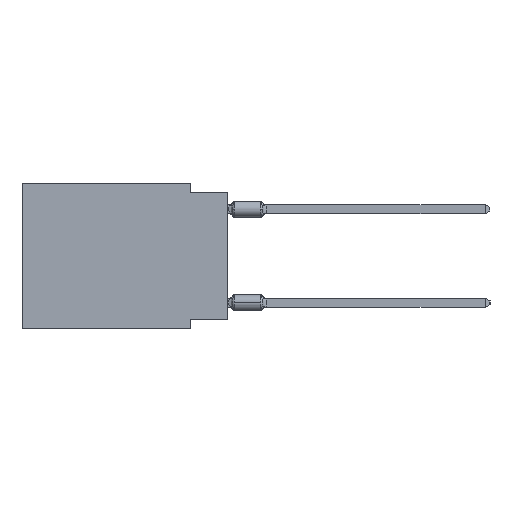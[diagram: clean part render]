
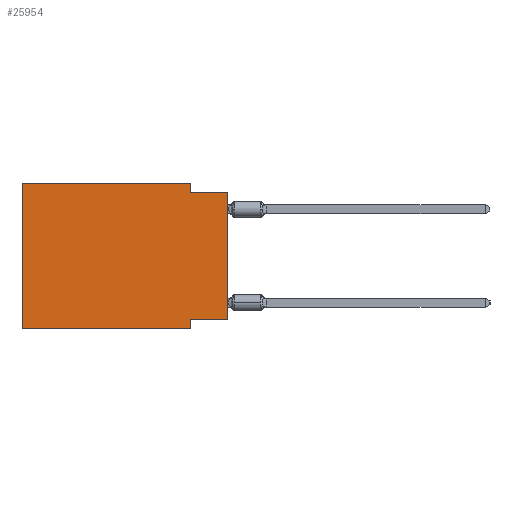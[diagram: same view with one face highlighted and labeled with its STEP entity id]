
A CAD part, left-side view. The second image highlights one B-rep face of the part: STEP entity #25954.
In plain terms, the highlighted planar face has unit normal (-1, 0, 0).
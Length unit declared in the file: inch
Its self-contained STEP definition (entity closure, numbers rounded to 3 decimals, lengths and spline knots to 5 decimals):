
#941 = ORIENTED_EDGE ( 'NONE', *, *, #7162, .T. ) ;
#1256 = EDGE_CURVE ( 'NONE', #4741, #25546, #44619, .T. ) ;
#1490 = LINE ( 'NONE', #14653, #12118 ) ;
#1783 = DIRECTION ( 'NONE',  ( 0., -1., 0. ) ) ;
#2938 = VECTOR ( 'NONE', #43295, 39.37008 ) ;
#3073 = LINE ( 'NONE', #11270, #56207 ) ;
#4071 = VERTEX_POINT ( 'NONE', #52990 ) ;
#4741 = VERTEX_POINT ( 'NONE', #26559 ) ;
#5107 = CARTESIAN_POINT ( 'NONE',  ( 0., 0.1, -0.025 ) ) ;
#7162 = EDGE_CURVE ( 'NONE', #4741, #17069, #37907, .T. ) ;
#7419 = CARTESIAN_POINT ( 'NONE',  ( 0., 0., -0.025 ) ) ;
#7439 = ORIENTED_EDGE ( 'NONE', *, *, #41969, .F. ) ;
#8390 = VECTOR ( 'NONE', #41917, 39.37008 ) ;
#10567 = LINE ( 'NONE', #11135, #43037 ) ;
#10847 = DIRECTION ( 'NONE',  ( 0., 0., 1. ) ) ;
#11135 = CARTESIAN_POINT ( 'NONE',  ( 0., 0., -0.365 ) ) ;
#11270 = CARTESIAN_POINT ( 'NONE',  ( 0., 0.55, 0. ) ) ;
#12118 = VECTOR ( 'NONE', #1783, 39.37008 ) ;
#12351 = CARTESIAN_POINT ( 'NONE',  ( 0., 0.1, -0.39 ) ) ;
#14587 = FACE_OUTER_BOUND ( 'NONE', #33785, .T. ) ;
#14653 = CARTESIAN_POINT ( 'NONE',  ( 0., 0., -0.025 ) ) ;
#15165 = CARTESIAN_POINT ( 'NONE',  ( 0., 0.55, 0. ) ) ;
#17069 = VERTEX_POINT ( 'NONE', #12351 ) ;
#20062 = ORIENTED_EDGE ( 'NONE', *, *, #33660, .T. ) ;
#20437 = LINE ( 'NONE', #38310, #2938 ) ;
#20591 = EDGE_CURVE ( 'NONE', #52373, #43440, #1490, .T. ) ;
#21162 = ORIENTED_EDGE ( 'NONE', *, *, #32842, .F. ) ;
#21853 = EDGE_CURVE ( 'NONE', #40993, #4071, #10567, .T. ) ;
#22333 = CARTESIAN_POINT ( 'NONE',  ( 0., 0.55, 0. ) ) ;
#24034 = LINE ( 'NONE', #37512, #8390 ) ;
#25017 = DIRECTION ( 'NONE',  ( 0., -1., 0. ) ) ;
#25546 = VERTEX_POINT ( 'NONE', #28119 ) ;
#25954 = ADVANCED_FACE ( 'NONE', ( #14587 ), #50323, .F. ) ;
#26559 = CARTESIAN_POINT ( 'NONE',  ( 0., 0.55, -0.39 ) ) ;
#28119 = CARTESIAN_POINT ( 'NONE',  ( 0., 0.55, 0. ) ) ;
#28281 = ORIENTED_EDGE ( 'NONE', *, *, #1256, .F. ) ;
#28833 = DIRECTION ( 'NONE',  ( 0., -1., 0. ) ) ;
#30978 = CARTESIAN_POINT ( 'NONE',  ( 0., 0., -0.365 ) ) ;
#32842 = EDGE_CURVE ( 'NONE', #25546, #52557, #3073, .T. ) ;
#33028 = DIRECTION ( 'NONE',  ( 1., 0., 0. ) ) ;
#33385 = CARTESIAN_POINT ( 'NONE',  ( 0., 0., 0. ) ) ;
#33660 = EDGE_CURVE ( 'NONE', #40993, #43440, #42461, .T. ) ;
#33785 = EDGE_LOOP ( 'NONE', ( #20062, #37670, #7439, #21162, #28281, #941, #42858, #34050 ) ) ;
#33812 = CARTESIAN_POINT ( 'NONE',  ( 0., 0.55, -0.39 ) ) ;
#33816 = VECTOR ( 'NONE', #10847, 39.37008 ) ;
#34050 = ORIENTED_EDGE ( 'NONE', *, *, #21853, .F. ) ;
#34061 = CARTESIAN_POINT ( 'NONE',  ( 0., 0.1, 0. ) ) ;
#34201 = VECTOR ( 'NONE', #25017, 39.37008 ) ;
#37512 = CARTESIAN_POINT ( 'NONE',  ( 0., 0.1, 0. ) ) ;
#37670 = ORIENTED_EDGE ( 'NONE', *, *, #20591, .F. ) ;
#37907 = LINE ( 'NONE', #33812, #34201 ) ;
#38310 = CARTESIAN_POINT ( 'NONE',  ( 0., 0.1, -0.39 ) ) ;
#40993 = VERTEX_POINT ( 'NONE', #30978 ) ;
#41917 = DIRECTION ( 'NONE',  ( 0., 0., -1. ) ) ;
#41969 = EDGE_CURVE ( 'NONE', #52557, #52373, #24034, .T. ) ;
#42461 = LINE ( 'NONE', #33385, #33816 ) ;
#42858 = ORIENTED_EDGE ( 'NONE', *, *, #46620, .F. ) ;
#43037 = VECTOR ( 'NONE', #46280, 39.37008 ) ;
#43295 = DIRECTION ( 'NONE',  ( 0., 0., -1. ) ) ;
#43440 = VERTEX_POINT ( 'NONE', #7419 ) ;
#44619 = LINE ( 'NONE', #22333, #56326 ) ;
#46280 = DIRECTION ( 'NONE',  ( 0., 1., 0. ) ) ;
#46506 = DIRECTION ( 'NONE',  ( 0., 0., -1. ) ) ;
#46620 = EDGE_CURVE ( 'NONE', #4071, #17069, #20437, .T. ) ;
#50323 = PLANE ( 'NONE',  #54845 ) ;
#52227 = DIRECTION ( 'NONE',  ( 0., 0., 1. ) ) ;
#52373 = VERTEX_POINT ( 'NONE', #5107 ) ;
#52557 = VERTEX_POINT ( 'NONE', #34061 ) ;
#52990 = CARTESIAN_POINT ( 'NONE',  ( 0., 0.1, -0.365 ) ) ;
#54845 = AXIS2_PLACEMENT_3D ( 'NONE', #15165, #33028, #46506 ) ;
#56207 = VECTOR ( 'NONE', #28833, 39.37008 ) ;
#56326 = VECTOR ( 'NONE', #52227, 39.37008 ) ;
